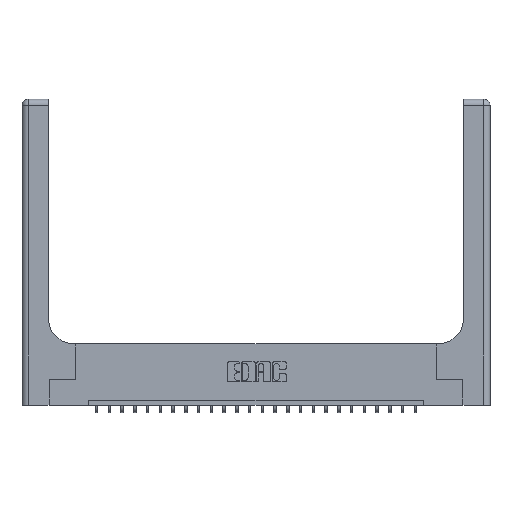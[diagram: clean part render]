
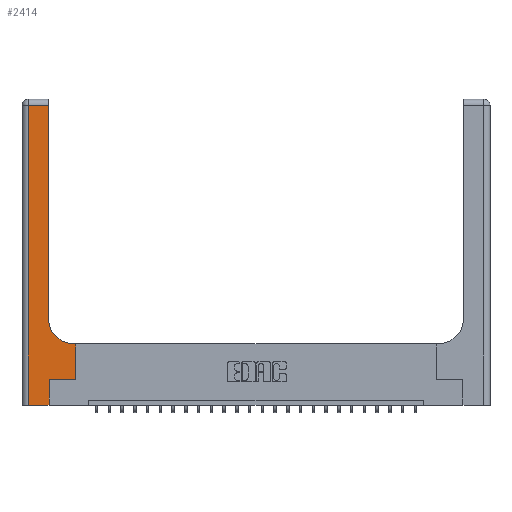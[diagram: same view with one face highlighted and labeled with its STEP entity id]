
A CAD part, top view. The second image highlights one B-rep face of the part: STEP entity #2414.
In plain terms, the highlighted planar face has unit normal (0, 0, 1).
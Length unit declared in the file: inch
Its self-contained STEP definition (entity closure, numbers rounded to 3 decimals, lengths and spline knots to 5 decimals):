
#1013 = FACE_OUTER_BOUND ( 'NONE', #10326, .T. ) ;
#1418 = DIRECTION ( 'NONE',  ( -1., 0., 0. ) ) ;
#2216 = CARTESIAN_POINT ( 'NONE',  ( 0.528, 0.6, 0.37 ) ) ;
#2414 = ADVANCED_FACE ( 'NONE', ( #1013 ), #8180, .F. ) ;
#2486 = CARTESIAN_POINT ( 'NONE',  ( 0.265, 0., 0.37 ) ) ;
#2518 = DIRECTION ( 'NONE',  ( -1., 0., 0. ) ) ;
#2831 = LINE ( 'NONE', #5136, #8282 ) ;
#3357 = CARTESIAN_POINT ( 'NONE',  ( 0.528, 0.25, 0.37 ) ) ;
#3583 = ORIENTED_EDGE ( 'NONE', *, *, #20518, .T. ) ;
#3841 = AXIS2_PLACEMENT_3D ( 'NONE', #21273, #10358, #9887 ) ;
#4027 = CARTESIAN_POINT ( 'NONE',  ( 0.06, 0., 0.37 ) ) ;
#4931 = VERTEX_POINT ( 'NONE', #2486 ) ;
#5063 = CARTESIAN_POINT ( 'NONE',  ( 0.26, 0.6, 0.37 ) ) ;
#5136 = CARTESIAN_POINT ( 'NONE',  ( 0., 0., 0.37 ) ) ;
#5411 = VERTEX_POINT ( 'NONE', #4027 ) ;
#5661 = CARTESIAN_POINT ( 'NONE',  ( 0.265, 0.25, 0.37 ) ) ;
#6321 = DIRECTION ( 'NONE',  ( 1., 0., 0. ) ) ;
#6487 = DIRECTION ( 'NONE',  ( 0., 1., 0. ) ) ;
#7008 = CARTESIAN_POINT ( 'NONE',  ( 0.06, 3., 0.37 ) ) ;
#7277 = ORIENTED_EDGE ( 'NONE', *, *, #19132, .T. ) ;
#7985 = CARTESIAN_POINT ( 'NONE',  ( 0., 2.94, 0.37 ) ) ;
#8063 = CARTESIAN_POINT ( 'NONE',  ( 0.265, 0., 0.37 ) ) ;
#8180 = PLANE ( 'NONE',  #3841 ) ;
#8282 = VECTOR ( 'NONE', #19929, 39.37008 ) ;
#8527 = LINE ( 'NONE', #10817, #9805 ) ;
#9463 = DIRECTION ( 'NONE',  ( 1., 0., 0. ) ) ;
#9805 = VECTOR ( 'NONE', #20391, 39.37008 ) ;
#9887 = DIRECTION ( 'NONE',  ( -1., 0., 0. ) ) ;
#10040 = EDGE_CURVE ( 'NONE', #18628, #22656, #13479, .T. ) ;
#10242 = LINE ( 'NONE', #8063, #10262 ) ;
#10262 = VECTOR ( 'NONE', #6487, 39.37008 ) ;
#10285 = EDGE_CURVE ( 'NONE', #12112, #15233, #21193, .T. ) ;
#10301 = CARTESIAN_POINT ( 'NONE',  ( 0.26, 0.85, 0.37 ) ) ;
#10326 = EDGE_LOOP ( 'NONE', ( #22347, #11495, #20663, #3583, #13467, #17037, #7277, #23450, #14844 ) ) ;
#10358 = DIRECTION ( 'NONE',  ( 0., 0., -1. ) ) ;
#10387 = VERTEX_POINT ( 'NONE', #2216 ) ;
#10396 = DIRECTION ( 'NONE',  ( 0., -1., 0. ) ) ;
#10817 = CARTESIAN_POINT ( 'NONE',  ( 0.26, 3., 0.37 ) ) ;
#11495 = ORIENTED_EDGE ( 'NONE', *, *, #10285, .T. ) ;
#12112 = VERTEX_POINT ( 'NONE', #13478 ) ;
#12558 = EDGE_CURVE ( 'NONE', #15702, #14096, #15371, .T. ) ;
#13467 = ORIENTED_EDGE ( 'NONE', *, *, #22208, .T. ) ;
#13478 = CARTESIAN_POINT ( 'NONE',  ( 0.26, 2.94, 0.37 ) ) ;
#13479 = CIRCLE ( 'NONE', #20074, 0.25 ) ;
#14056 = EDGE_CURVE ( 'NONE', #15233, #5411, #17409, .T. ) ;
#14096 = VERTEX_POINT ( 'NONE', #3357 ) ;
#14762 = CARTESIAN_POINT ( 'NONE',  ( 0.06, 2.94, 0.37 ) ) ;
#14844 = ORIENTED_EDGE ( 'NONE', *, *, #10040, .T. ) ;
#15233 = VERTEX_POINT ( 'NONE', #14762 ) ;
#15310 = DIRECTION ( 'NONE',  ( 0., 1., 0. ) ) ;
#15371 = LINE ( 'NONE', #22791, #22440 ) ;
#15489 = EDGE_CURVE ( 'NONE', #10387, #18628, #17668, .T. ) ;
#15702 = VERTEX_POINT ( 'NONE', #5661 ) ;
#17028 = VECTOR ( 'NONE', #10396, 39.37008 ) ;
#17037 = ORIENTED_EDGE ( 'NONE', *, *, #12558, .T. ) ;
#17409 = LINE ( 'NONE', #7008, #17028 ) ;
#17548 = EDGE_CURVE ( 'NONE', #22656, #12112, #8527, .T. ) ;
#17668 = LINE ( 'NONE', #5063, #22521 ) ;
#18628 = VERTEX_POINT ( 'NONE', #22291 ) ;
#18902 = VECTOR ( 'NONE', #2518, 39.37008 ) ;
#19132 = EDGE_CURVE ( 'NONE', #14096, #10387, #23720, .T. ) ;
#19929 = DIRECTION ( 'NONE',  ( 1., 0., 0. ) ) ;
#20074 = AXIS2_PLACEMENT_3D ( 'NONE', #22702, #20752, #6321 ) ;
#20391 = DIRECTION ( 'NONE',  ( 0., 1., 0. ) ) ;
#20518 = EDGE_CURVE ( 'NONE', #5411, #4931, #2831, .T. ) ;
#20663 = ORIENTED_EDGE ( 'NONE', *, *, #14056, .T. ) ;
#20696 = VECTOR ( 'NONE', #15310, 39.37008 ) ;
#20752 = DIRECTION ( 'NONE',  ( 0., 0., -1. ) ) ;
#21193 = LINE ( 'NONE', #7985, #18902 ) ;
#21273 = CARTESIAN_POINT ( 'NONE',  ( 0., 3., 0.37 ) ) ;
#22208 = EDGE_CURVE ( 'NONE', #4931, #15702, #10242, .T. ) ;
#22291 = CARTESIAN_POINT ( 'NONE',  ( 0.51, 0.6, 0.37 ) ) ;
#22347 = ORIENTED_EDGE ( 'NONE', *, *, #17548, .T. ) ;
#22440 = VECTOR ( 'NONE', #9463, 39.37008 ) ;
#22521 = VECTOR ( 'NONE', #1418, 39.37008 ) ;
#22656 = VERTEX_POINT ( 'NONE', #10301 ) ;
#22702 = CARTESIAN_POINT ( 'NONE',  ( 0.51, 0.85, 0.37 ) ) ;
#22791 = CARTESIAN_POINT ( 'NONE',  ( 0.265, 0.25, 0.37 ) ) ;
#22973 = CARTESIAN_POINT ( 'NONE',  ( 0.528, 0.25, 0.37 ) ) ;
#23450 = ORIENTED_EDGE ( 'NONE', *, *, #15489, .T. ) ;
#23720 = LINE ( 'NONE', #22973, #20696 ) ;
